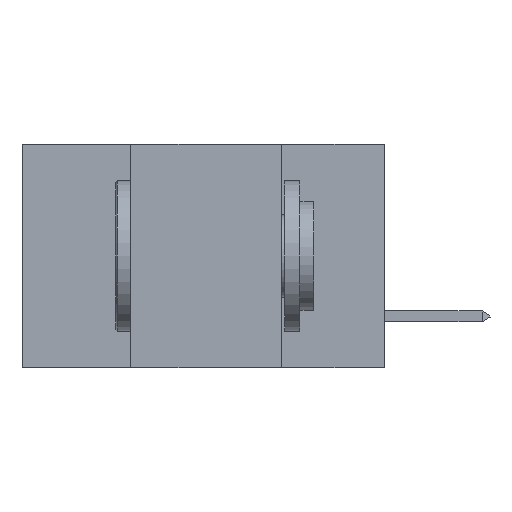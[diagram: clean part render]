
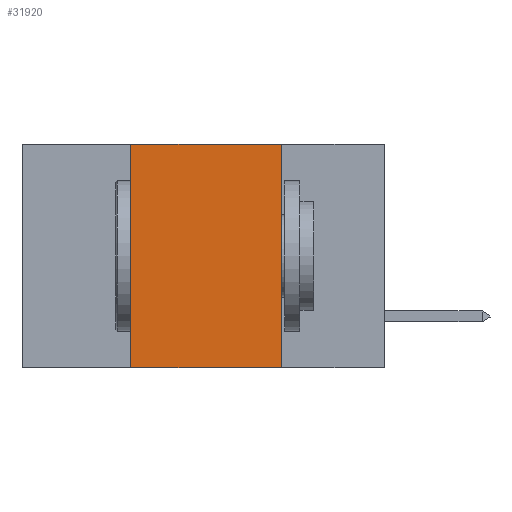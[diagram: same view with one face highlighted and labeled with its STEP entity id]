
A CAD part, left-side view. The second image highlights one B-rep face of the part: STEP entity #31920.
In plain terms, the highlighted planar face has unit normal (-1, 0, 0).
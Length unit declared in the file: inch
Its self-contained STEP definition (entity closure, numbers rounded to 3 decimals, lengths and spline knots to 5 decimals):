
#2093 = CARTESIAN_POINT ( 'NONE',  ( 0., 0.42, 0. ) ) ;
#2374 = EDGE_LOOP ( 'NONE', ( #46172, #33906, #43386, #22993 ) ) ;
#2946 = DIRECTION ( 'NONE',  ( 0., -1., 0. ) ) ;
#4327 = CARTESIAN_POINT ( 'NONE',  ( 0., 0.42, -0.37 ) ) ;
#6425 = DIRECTION ( 'NONE',  ( 1., 0., 0. ) ) ;
#8660 = LINE ( 'NONE', #2093, #28041 ) ;
#9721 = FACE_OUTER_BOUND ( 'NONE', #2374, .T. ) ;
#13901 = DIRECTION ( 'NONE',  ( 0., 0., -1. ) ) ;
#15634 = VECTOR ( 'NONE', #17526, 39.37008 ) ;
#17451 = VERTEX_POINT ( 'NONE', #4327 ) ;
#17496 = LINE ( 'NONE', #39723, #15634 ) ;
#17526 = DIRECTION ( 'NONE',  ( 0., 0., -1. ) ) ;
#17631 = DIRECTION ( 'NONE',  ( 0., 0., 1. ) ) ;
#17702 = CARTESIAN_POINT ( 'NONE',  ( 0., 0.6, 0. ) ) ;
#18506 = VERTEX_POINT ( 'NONE', #31109 ) ;
#20164 = EDGE_CURVE ( 'NONE', #17451, #18506, #28545, .T. ) ;
#22993 = ORIENTED_EDGE ( 'NONE', *, *, #20164, .T. ) ;
#23767 = VECTOR ( 'NONE', #39535, 39.37008 ) ;
#25789 = CARTESIAN_POINT ( 'NONE',  ( 0., 0.17, 0. ) ) ;
#28041 = VECTOR ( 'NONE', #17631, 39.37008 ) ;
#28545 = LINE ( 'NONE', #28656, #33777 ) ;
#28656 = CARTESIAN_POINT ( 'NONE',  ( 0., 0.6, -0.37 ) ) ;
#29344 = PLANE ( 'NONE',  #43874 ) ;
#31109 = CARTESIAN_POINT ( 'NONE',  ( 0., 0.17, -0.37 ) ) ;
#31537 = CARTESIAN_POINT ( 'NONE',  ( 0., 0.42, 0. ) ) ;
#31920 = ADVANCED_FACE ( 'NONE', ( #9721 ), #29344, .F. ) ;
#33777 = VECTOR ( 'NONE', #2946, 39.37008 ) ;
#33906 = ORIENTED_EDGE ( 'NONE', *, *, #39828, .F. ) ;
#34570 = VERTEX_POINT ( 'NONE', #31537 ) ;
#36275 = VERTEX_POINT ( 'NONE', #25789 ) ;
#39535 = DIRECTION ( 'NONE',  ( 0., -1., 0. ) ) ;
#39723 = CARTESIAN_POINT ( 'NONE',  ( 0., 0.17, 0. ) ) ;
#39828 = EDGE_CURVE ( 'NONE', #34570, #36275, #43852, .T. ) ;
#43386 = ORIENTED_EDGE ( 'NONE', *, *, #44587, .F. ) ;
#43852 = LINE ( 'NONE', #47400, #23767 ) ;
#43874 = AXIS2_PLACEMENT_3D ( 'NONE', #17702, #6425, #13901 ) ;
#44587 = EDGE_CURVE ( 'NONE', #17451, #34570, #8660, .T. ) ;
#44718 = EDGE_CURVE ( 'NONE', #36275, #18506, #17496, .T. ) ;
#46172 = ORIENTED_EDGE ( 'NONE', *, *, #44718, .F. ) ;
#47400 = CARTESIAN_POINT ( 'NONE',  ( 0., 0.6, 0. ) ) ;
